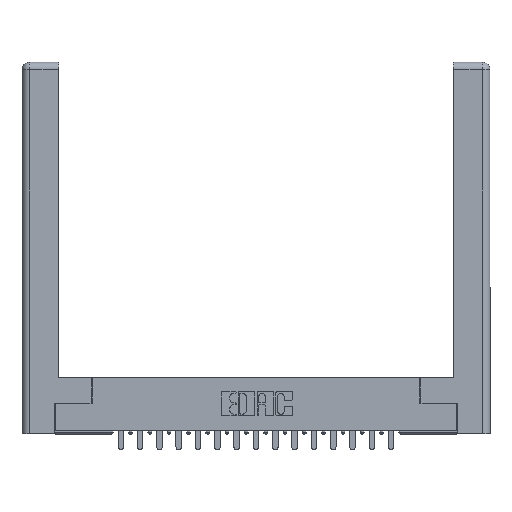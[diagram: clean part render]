
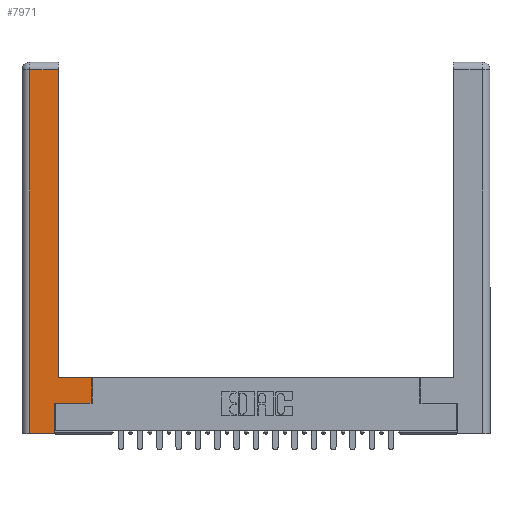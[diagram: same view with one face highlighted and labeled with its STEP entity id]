
A CAD part, top view. The second image highlights one B-rep face of the part: STEP entity #7971.
In plain terms, the highlighted planar face has unit normal (0, 0, 1).
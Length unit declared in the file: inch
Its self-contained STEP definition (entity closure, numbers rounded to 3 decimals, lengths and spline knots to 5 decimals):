
#217 = DIRECTION ( 'NONE',  ( 0., 1., 0. ) ) ;
#391 = FACE_OUTER_BOUND ( 'NONE', #12277, .T. ) ;
#645 = CARTESIAN_POINT ( 'NONE',  ( 0.0615, 2.94, 0. ) ) ;
#705 = CARTESIAN_POINT ( 'NONE',  ( 0.0615, 0., 0. ) ) ;
#752 = ORIENTED_EDGE ( 'NONE', *, *, #10938, .T. ) ;
#1293 = LINE ( 'NONE', #19620, #15929 ) ;
#1944 = VERTEX_POINT ( 'NONE', #705 ) ;
#2052 = CARTESIAN_POINT ( 'NONE',  ( 0.565, 0.45, 0. ) ) ;
#2253 = CARTESIAN_POINT ( 'NONE',  ( 0.295, 0.45, 0. ) ) ;
#2326 = VERTEX_POINT ( 'NONE', #2253 ) ;
#2824 = EDGE_CURVE ( 'NONE', #14682, #15536, #19686, .T. ) ;
#3185 = DIRECTION ( 'NONE',  ( 1., 0., 0. ) ) ;
#3658 = EDGE_CURVE ( 'NONE', #2326, #14627, #5654, .T. ) ;
#3715 = CARTESIAN_POINT ( 'NONE',  ( 0.265, 0.245, 0. ) ) ;
#4170 = DIRECTION ( 'NONE',  ( -1., 0., 0. ) ) ;
#4431 = LINE ( 'NONE', #645, #12912 ) ;
#4676 = ORIENTED_EDGE ( 'NONE', *, *, #6035, .T. ) ;
#4788 = VERTEX_POINT ( 'NONE', #19558 ) ;
#4989 = ORIENTED_EDGE ( 'NONE', *, *, #14039, .T. ) ;
#5222 = VECTOR ( 'NONE', #4170, 39.37008 ) ;
#5344 = VERTEX_POINT ( 'NONE', #6058 ) ;
#5654 = LINE ( 'NONE', #11036, #8295 ) ;
#6035 = EDGE_CURVE ( 'NONE', #1944, #14682, #12981, .T. ) ;
#6058 = CARTESIAN_POINT ( 'NONE',  ( 0.565, 0.45, 0. ) ) ;
#6516 = DIRECTION ( 'NONE',  ( 1., 0., 0. ) ) ;
#6718 = DIRECTION ( 'NONE',  ( -1., 0., 0. ) ) ;
#6866 = VECTOR ( 'NONE', #3185, 39.37008 ) ;
#6867 = CARTESIAN_POINT ( 'NONE',  ( 0., 0., 0. ) ) ;
#7338 = EDGE_CURVE ( 'NONE', #5344, #2326, #17186, .T. ) ;
#7971 = ADVANCED_FACE ( 'NONE', ( #391 ), #16328, .F. ) ;
#8295 = VECTOR ( 'NONE', #17903, 39.37008 ) ;
#8346 = VERTEX_POINT ( 'NONE', #17640 ) ;
#8675 = CARTESIAN_POINT ( 'NONE',  ( 0.295, 2.94, 0. ) ) ;
#8886 = DIRECTION ( 'NONE',  ( 0., 1., 0. ) ) ;
#8968 = ORIENTED_EDGE ( 'NONE', *, *, #7338, .T. ) ;
#9501 = ORIENTED_EDGE ( 'NONE', *, *, #13041, .T. ) ;
#9887 = ORIENTED_EDGE ( 'NONE', *, *, #19031, .T. ) ;
#10315 = VECTOR ( 'NONE', #217, 39.37008 ) ;
#10855 = CARTESIAN_POINT ( 'NONE',  ( 0.295, 0.45, 0. ) ) ;
#10938 = EDGE_CURVE ( 'NONE', #14627, #8346, #4431, .T. ) ;
#11036 = CARTESIAN_POINT ( 'NONE',  ( 0.295, 3., 0. ) ) ;
#12277 = EDGE_LOOP ( 'NONE', ( #12474, #752, #4989, #4676, #13554, #9887, #9501, #8968 ) ) ;
#12474 = ORIENTED_EDGE ( 'NONE', *, *, #3658, .T. ) ;
#12912 = VECTOR ( 'NONE', #17749, 39.37008 ) ;
#12981 = LINE ( 'NONE', #21795, #6866 ) ;
#13041 = EDGE_CURVE ( 'NONE', #4788, #5344, #14938, .T. ) ;
#13554 = ORIENTED_EDGE ( 'NONE', *, *, #2824, .T. ) ;
#13666 = DIRECTION ( 'NONE',  ( 0., 0., -1. ) ) ;
#13937 = CARTESIAN_POINT ( 'NONE',  ( 0.265, 0., 0. ) ) ;
#14039 = EDGE_CURVE ( 'NONE', #8346, #1944, #15984, .T. ) ;
#14627 = VERTEX_POINT ( 'NONE', #8675 ) ;
#14682 = VERTEX_POINT ( 'NONE', #13937 ) ;
#14938 = LINE ( 'NONE', #2052, #17877 ) ;
#15536 = VERTEX_POINT ( 'NONE', #3715 ) ;
#15929 = VECTOR ( 'NONE', #6516, 39.37008 ) ;
#15984 = LINE ( 'NONE', #19407, #19737 ) ;
#16328 = PLANE ( 'NONE',  #21611 ) ;
#17186 = LINE ( 'NONE', #10855, #5222 ) ;
#17640 = CARTESIAN_POINT ( 'NONE',  ( 0.0615, 2.94, 0. ) ) ;
#17749 = DIRECTION ( 'NONE',  ( -1., 0., 0. ) ) ;
#17877 = VECTOR ( 'NONE', #8886, 39.37008 ) ;
#17887 = DIRECTION ( 'NONE',  ( 0., -1., 0. ) ) ;
#17903 = DIRECTION ( 'NONE',  ( 0., 1., 0. ) ) ;
#18842 = CARTESIAN_POINT ( 'NONE',  ( 0.265, 0.245, 0. ) ) ;
#19031 = EDGE_CURVE ( 'NONE', #15536, #4788, #1293, .T. ) ;
#19407 = CARTESIAN_POINT ( 'NONE',  ( 0.0615, 0., 0. ) ) ;
#19558 = CARTESIAN_POINT ( 'NONE',  ( 0.565, 0.245, 0. ) ) ;
#19620 = CARTESIAN_POINT ( 'NONE',  ( 0.565, 0.245, 0. ) ) ;
#19686 = LINE ( 'NONE', #18842, #10315 ) ;
#19737 = VECTOR ( 'NONE', #17887, 39.37008 ) ;
#21611 = AXIS2_PLACEMENT_3D ( 'NONE', #6867, #13666, #6718 ) ;
#21795 = CARTESIAN_POINT ( 'NONE',  ( 0.265, 0., 0. ) ) ;
